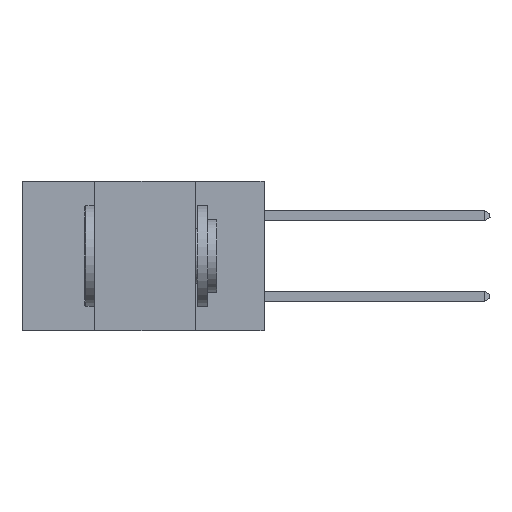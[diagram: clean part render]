
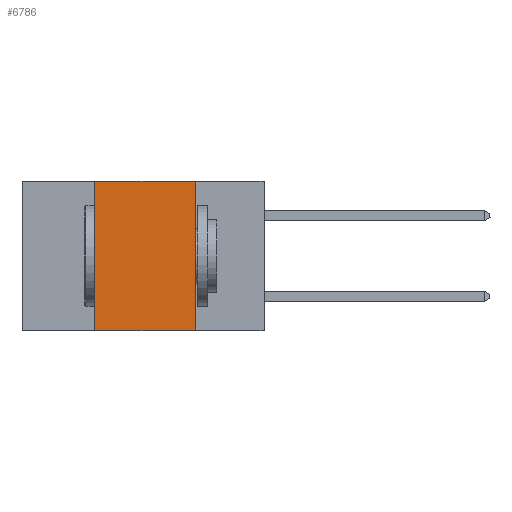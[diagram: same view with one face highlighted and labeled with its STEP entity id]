
A CAD part, left-side view. The second image highlights one B-rep face of the part: STEP entity #6786.
In plain terms, the highlighted planar face has unit normal (-1, 0, 0).
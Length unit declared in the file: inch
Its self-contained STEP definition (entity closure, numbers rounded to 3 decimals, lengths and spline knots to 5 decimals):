
#239 = LINE ( 'NONE', #10976, #8104 ) ;
#314 = EDGE_CURVE ( 'NONE', #19616, #5002, #2367, .T. ) ;
#843 = EDGE_CURVE ( 'NONE', #14631, #19616, #11427, .T. ) ;
#1181 = VERTEX_POINT ( 'NONE', #11568 ) ;
#1537 = CARTESIAN_POINT ( 'NONE',  ( 0., 0.6, 0. ) ) ;
#2367 = LINE ( 'NONE', #1537, #13247 ) ;
#2918 = EDGE_LOOP ( 'NONE', ( #17343, #15048, #3940, #16195 ) ) ;
#3161 = DIRECTION ( 'NONE',  ( 1., 0., 0. ) ) ;
#3940 = ORIENTED_EDGE ( 'NONE', *, *, #843, .F. ) ;
#5002 = VERTEX_POINT ( 'NONE', #23137 ) ;
#5769 = FACE_OUTER_BOUND ( 'NONE', #2918, .T. ) ;
#6130 = DIRECTION ( 'NONE',  ( 0., 0., 1. ) ) ;
#6284 = VECTOR ( 'NONE', #6130, 39.37008 ) ;
#6462 = LINE ( 'NONE', #18970, #10985 ) ;
#6786 = ADVANCED_FACE ( 'NONE', ( #5769 ), #22051, .F. ) ;
#8104 = VECTOR ( 'NONE', #24457, 39.37008 ) ;
#8560 = AXIS2_PLACEMENT_3D ( 'NONE', #24322, #3161, #14465 ) ;
#9546 = DIRECTION ( 'NONE',  ( 0., -1., 0. ) ) ;
#10976 = CARTESIAN_POINT ( 'NONE',  ( 0., 0.6, -0.37 ) ) ;
#10985 = VECTOR ( 'NONE', #22780, 39.37008 ) ;
#11427 = LINE ( 'NONE', #23645, #6284 ) ;
#11446 = EDGE_CURVE ( 'NONE', #5002, #1181, #6462, .T. ) ;
#11568 = CARTESIAN_POINT ( 'NONE',  ( 0., 0.17, -0.37 ) ) ;
#13247 = VECTOR ( 'NONE', #9546, 39.37008 ) ;
#14465 = DIRECTION ( 'NONE',  ( 0., 0., -1. ) ) ;
#14631 = VERTEX_POINT ( 'NONE', #24815 ) ;
#15048 = ORIENTED_EDGE ( 'NONE', *, *, #314, .F. ) ;
#16195 = ORIENTED_EDGE ( 'NONE', *, *, #18627, .T. ) ;
#17343 = ORIENTED_EDGE ( 'NONE', *, *, #11446, .F. ) ;
#18627 = EDGE_CURVE ( 'NONE', #14631, #1181, #239, .T. ) ;
#18970 = CARTESIAN_POINT ( 'NONE',  ( 0., 0.17, 0. ) ) ;
#19616 = VERTEX_POINT ( 'NONE', #24293 ) ;
#22051 = PLANE ( 'NONE',  #8560 ) ;
#22780 = DIRECTION ( 'NONE',  ( 0., 0., -1. ) ) ;
#23137 = CARTESIAN_POINT ( 'NONE',  ( 0., 0.17, 0. ) ) ;
#23645 = CARTESIAN_POINT ( 'NONE',  ( 0., 0.42, 0. ) ) ;
#24293 = CARTESIAN_POINT ( 'NONE',  ( 0., 0.42, 0. ) ) ;
#24322 = CARTESIAN_POINT ( 'NONE',  ( 0., 0.6, 0. ) ) ;
#24457 = DIRECTION ( 'NONE',  ( 0., -1., 0. ) ) ;
#24815 = CARTESIAN_POINT ( 'NONE',  ( 0., 0.42, -0.37 ) ) ;
